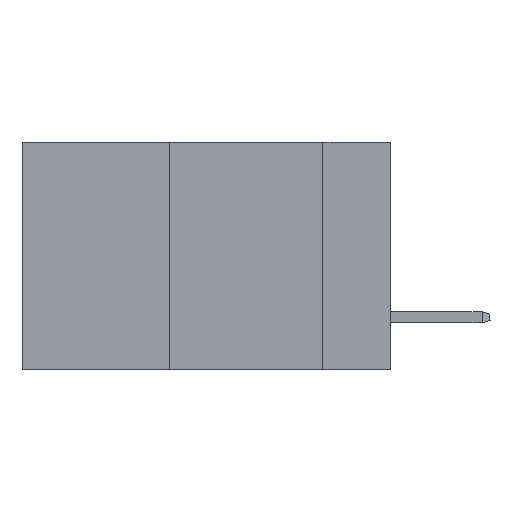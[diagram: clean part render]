
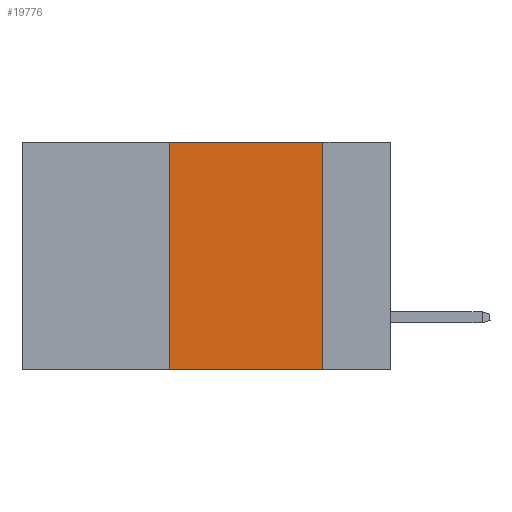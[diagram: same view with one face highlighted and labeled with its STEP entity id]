
A CAD part, left-side view. The second image highlights one B-rep face of the part: STEP entity #19776.
In plain terms, the highlighted planar face has unit normal (-1, 0, 0).
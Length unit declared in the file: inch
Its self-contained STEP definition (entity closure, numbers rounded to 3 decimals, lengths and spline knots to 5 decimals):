
#545 = CARTESIAN_POINT ( 'NONE',  ( 0., 0.36, 0. ) ) ;
#549 = EDGE_CURVE ( 'NONE', #22546, #1437, #13463, .T. ) ;
#1437 = VERTEX_POINT ( 'NONE', #5602 ) ;
#1923 = CARTESIAN_POINT ( 'NONE',  ( 0., 0.6, 0. ) ) ;
#2721 = AXIS2_PLACEMENT_3D ( 'NONE', #15393, #3252, #17434 ) ;
#2887 = ORIENTED_EDGE ( 'NONE', *, *, #14180, .F. ) ;
#3252 = DIRECTION ( 'NONE',  ( 1., 0., 0. ) ) ;
#5602 = CARTESIAN_POINT ( 'NONE',  ( 0., 0.11, 0. ) ) ;
#6146 = LINE ( 'NONE', #12354, #24223 ) ;
#6749 = DIRECTION ( 'NONE',  ( 0., 0., 1. ) ) ;
#7050 = PLANE ( 'NONE',  #2721 ) ;
#7159 = ORIENTED_EDGE ( 'NONE', *, *, #549, .F. ) ;
#9279 = FACE_OUTER_BOUND ( 'NONE', #22816, .T. ) ;
#9374 = EDGE_CURVE ( 'NONE', #1437, #19533, #26228, .T. ) ;
#10550 = LINE ( 'NONE', #545, #15286 ) ;
#11004 = DIRECTION ( 'NONE',  ( 0., 0., -1. ) ) ;
#12354 = CARTESIAN_POINT ( 'NONE',  ( 0., 0.6, -0.37 ) ) ;
#12594 = VECTOR ( 'NONE', #11004, 39.37008 ) ;
#12817 = VECTOR ( 'NONE', #20149, 39.37008 ) ;
#13463 = LINE ( 'NONE', #1923, #12817 ) ;
#14180 = EDGE_CURVE ( 'NONE', #20024, #22546, #10550, .T. ) ;
#15286 = VECTOR ( 'NONE', #6749, 39.37008 ) ;
#15393 = CARTESIAN_POINT ( 'NONE',  ( 0., 0.6, 0. ) ) ;
#16022 = DIRECTION ( 'NONE',  ( 0., -1., 0. ) ) ;
#17434 = DIRECTION ( 'NONE',  ( 0., 0., -1. ) ) ;
#17624 = CARTESIAN_POINT ( 'NONE',  ( 0., 0.36, 0. ) ) ;
#18117 = CARTESIAN_POINT ( 'NONE',  ( 0., 0.11, -0.37 ) ) ;
#19056 = CARTESIAN_POINT ( 'NONE',  ( 0., 0.11, 0. ) ) ;
#19533 = VERTEX_POINT ( 'NONE', #18117 ) ;
#19776 = ADVANCED_FACE ( 'NONE', ( #9279 ), #7050, .F. ) ;
#20024 = VERTEX_POINT ( 'NONE', #25574 ) ;
#20149 = DIRECTION ( 'NONE',  ( 0., -1., 0. ) ) ;
#20786 = EDGE_CURVE ( 'NONE', #20024, #19533, #6146, .T. ) ;
#22546 = VERTEX_POINT ( 'NONE', #17624 ) ;
#22816 = EDGE_LOOP ( 'NONE', ( #26162, #7159, #2887, #25123 ) ) ;
#24223 = VECTOR ( 'NONE', #16022, 39.37008 ) ;
#25123 = ORIENTED_EDGE ( 'NONE', *, *, #20786, .T. ) ;
#25574 = CARTESIAN_POINT ( 'NONE',  ( 0., 0.36, -0.37 ) ) ;
#26162 = ORIENTED_EDGE ( 'NONE', *, *, #9374, .F. ) ;
#26228 = LINE ( 'NONE', #19056, #12594 ) ;
